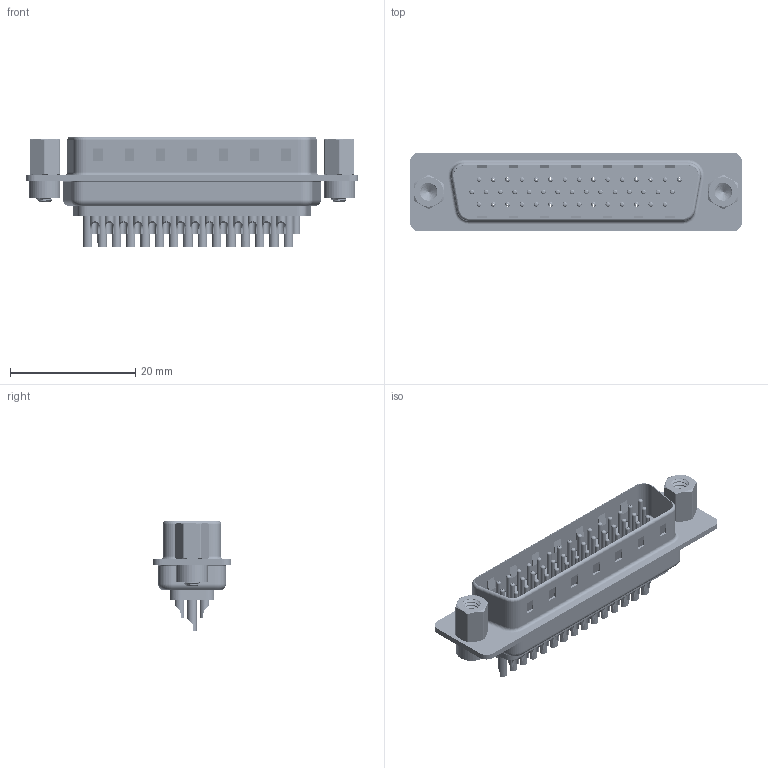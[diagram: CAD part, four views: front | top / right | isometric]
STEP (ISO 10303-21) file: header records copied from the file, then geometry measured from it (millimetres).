
FILE_DESCRIPTION (( 'STEP AP203' ), '1' );
FILE_NAME ('637-044-632-043.STEP', '2020-07-18T03:04:56', ( '' ), ( '' ), 'SwSTEP 2.0', 'SolidWorks 2020', '' );
FILE_SCHEMA (( 'CONFIG_CONTROL_DESIGN' ));
Length unit declared in the file: millimetre
Products named in the file (9): 637 4-40 Threaded Rivet; 637 Shell Front_44 Contacts; 637 Shell Rear_44 Contacts; 637 Contact Row 2_32; 637 Contact Row 3_32; 637-044-632-043; 637 4-40 Hex Standoff; 637 Contact Row 1_32; 637 Housing_44 Contacts
Assembly tree (51 placements, depth 2):
  637-044-632-043
    637 Housing_44 Contacts
    637 Shell Front_44 Contacts
    637 Shell Rear_44 Contacts
    637 Contact Row 1_32  x15
    637 Contact Row 2_32  x15
    637 Contact Row 3_32  x14
    637 4-40 Threaded Rivet  x2
    637 4-40 Hex Standoff  x2
Bounding box: 53 x 12.6 x 17.55 mm (x, y, z)
Volume: 2926.6 mm3; surface area: 10914.1 mm2
Topology: 51 solids, 51 shells, 3318 faces, 8521 edges, 5404 vertices
Faces by surface type: cylinder 1485, torus 974, plane 809, cone 32, bspline 18
Entity records: 34300 total; most frequent: CARTESIAN_POINT 9274, DIRECTION 5145, ORIENTED_EDGE 4556, EDGE_CURVE 2278, AXIS2_PLACEMENT_3D 2070, VERTEX_POINT 1467, EDGE_LOOP 1155, CIRCLE 1099
